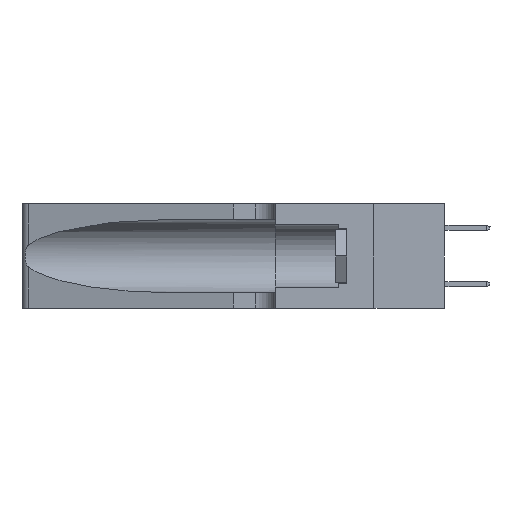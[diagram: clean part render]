
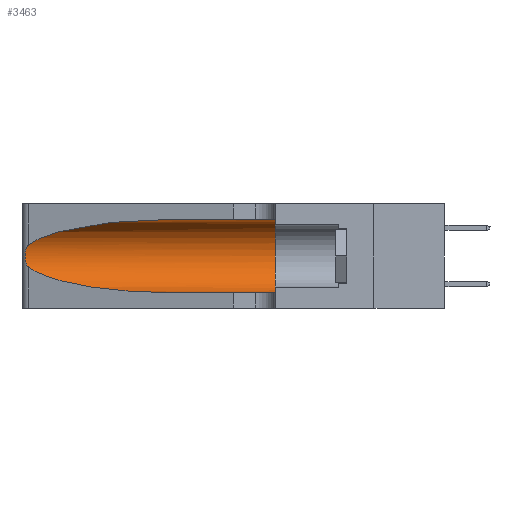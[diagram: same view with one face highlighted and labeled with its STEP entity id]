
A CAD part, left-side view. The second image highlights one B-rep face of the part: STEP entity #3463.
In plain terms, the highlighted cylindrical face has radius 3.308 mm (diameter 6.617 mm), a partial arc.
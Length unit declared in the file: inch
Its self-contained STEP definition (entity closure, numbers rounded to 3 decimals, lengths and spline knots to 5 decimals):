
#256 = CARTESIAN_POINT ( 'NONE',  ( 0.1305, 1.61858, 0.31525 ) ) ;
#488 = VERTEX_POINT ( 'NONE', #8735 ) ;
#558 = DIRECTION ( 'NONE',  ( 0., 0., -1. ) ) ;
#919 = CARTESIAN_POINT ( 'NONE',  ( 0.25639, 1.23184, 0.21858 ) ) ;
#1046 = CARTESIAN_POINT ( 'NONE',  ( 0.26017, 1.23833, 0.17102 ) ) ;
#1629 = DIRECTION ( 'NONE',  ( 0., 1., 0. ) ) ;
#1738 = CARTESIAN_POINT ( 'NONE',  ( 0.1305, 0.72297, 0.05475 ) ) ;
#2156 = CARTESIAN_POINT ( 'NONE',  ( 0.18966, 0.96281, 0.05475 ) ) ;
#2170 = ORIENTED_EDGE ( 'NONE', *, *, #7183, .T. ) ;
#2276 = CARTESIAN_POINT ( 'NONE',  ( 0.25789, 1.23486, 0.15765 ) ) ;
#2587 = VECTOR ( 'NONE', #6067, 39.37008 ) ;
#2995 = CARTESIAN_POINT ( 'NONE',  ( 0.25487, 1.22718, 0.22369 ) ) ;
#3277 = VECTOR ( 'NONE', #17913, 39.37008 ) ;
#3463 = ADVANCED_FACE ( 'NONE', ( #11032 ), #7582, .F. ) ;
#3469 = ORIENTED_EDGE ( 'NONE', *, *, #18091, .T. ) ;
#3883 = CARTESIAN_POINT ( 'NONE',  ( 0.25639, 1.23186, 0.15144 ) ) ;
#4797 = AXIS2_PLACEMENT_3D ( 'NONE', #17805, #1629, #17873 ) ;
#5348 = LINE ( 'NONE', #14806, #2587 ) ;
#6005 = LINE ( 'NONE', #256, #3277 ) ;
#6067 = DIRECTION ( 'NONE',  ( 0., -1., 0. ) ) ;
#6241 = EDGE_LOOP ( 'NONE', ( #17722, #2170, #3469, #12455, #13920, #12567 ) ) ;
#6276 = CARTESIAN_POINT ( 'NONE',  ( 0.1305, 1.61858, 0.185 ) ) ;
#6574 = CARTESIAN_POINT ( 'NONE',  ( 0.1305, 0.72297, 0.05475 ) ) ;
#6628 = CARTESIAN_POINT ( 'NONE',  ( 0.26018, 1.23835, 0.19895 ) ) ;
#6645 = VERTEX_POINT ( 'NONE', #17974 ) ;
#6747 = CARTESIAN_POINT ( 'NONE',  ( 0.25854, 1.2359, 0.20912 ) ) ;
#7183 = EDGE_CURVE ( 'NONE', #8647, #6645, #15826, .T. ) ;
#7582 = CYLINDRICAL_SURFACE ( 'NONE', #13383, 0.13025 ) ;
#7894 = EDGE_CURVE ( 'NONE', #15827, #8647, #16660, .T. ) ;
#8082 = CARTESIAN_POINT ( 'NONE',  ( 0.25487, 1.22718, 0.22369 ) ) ;
#8459 = CARTESIAN_POINT ( 'NONE',  ( 0.18966, 0.96281, 0.31525 ) ) ;
#8647 = VERTEX_POINT ( 'NONE', #2995 ) ;
#8735 = CARTESIAN_POINT ( 'NONE',  ( 0.1305, 0.35, 0.05475 ) ) ;
#8781 =( BOUNDED_CURVE ( )  B_SPLINE_CURVE ( 3, ( #12765, #17136, #2156, #6574 ),
 .UNSPECIFIED., .F., .F. ) 
 B_SPLINE_CURVE_WITH_KNOTS ( ( 4, 4 ),
 ( 3.44316, 4.71239 ),
 .UNSPECIFIED. ) 
 CURVE ( )  GEOMETRIC_REPRESENTATION_ITEM ( )  RATIONAL_B_SPLINE_CURVE ( ( 1., 0.87, 0.87, 1. ) ) 
 REPRESENTATION_ITEM ( '' )  );
#9706 = EDGE_CURVE ( 'NONE', #15827, #12617, #6005, .T. ) ;
#9782 = CARTESIAN_POINT ( 'NONE',  ( 0.1305, 0.72297, 0.31525 ) ) ;
#9786 = CARTESIAN_POINT ( 'NONE',  ( 0.25487, 1.22718, 0.14631 ) ) ;
#11032 = FACE_OUTER_BOUND ( 'NONE', #6241, .T. ) ;
#11165 = CARTESIAN_POINT ( 'NONE',  ( 0.25856, 1.23593, 0.16098 ) ) ;
#11533 = CARTESIAN_POINT ( 'NONE',  ( 0.2373, 1.15595, 0.28018 ) ) ;
#12455 = ORIENTED_EDGE ( 'NONE', *, *, #15504, .T. ) ;
#12567 = ORIENTED_EDGE ( 'NONE', *, *, #9706, .F. ) ;
#12617 = VERTEX_POINT ( 'NONE', #13093 ) ;
#12765 = CARTESIAN_POINT ( 'NONE',  ( 0.25487, 1.22718, 0.14631 ) ) ;
#13093 = CARTESIAN_POINT ( 'NONE',  ( 0.1305, 0.35, 0.31525 ) ) ;
#13171 = EDGE_CURVE ( 'NONE', #12617, #488, #18221, .T. ) ;
#13383 = AXIS2_PLACEMENT_3D ( 'NONE', #6276, #16561, #558 ) ;
#13920 = ORIENTED_EDGE ( 'NONE', *, *, #13171, .F. ) ;
#14806 = CARTESIAN_POINT ( 'NONE',  ( 0.1305, 1.61858, 0.05475 ) ) ;
#15211 = VERTEX_POINT ( 'NONE', #1738 ) ;
#15376 = CARTESIAN_POINT ( 'NONE',  ( 0.25555, 1.22994, 0.2215 ) ) ;
#15503 = CARTESIAN_POINT ( 'NONE',  ( 0.25787, 1.23484, 0.2124 ) ) ;
#15504 = EDGE_CURVE ( 'NONE', #15211, #488, #5348, .T. ) ;
#15826 = B_SPLINE_CURVE_WITH_KNOTS ( 'NONE', 3,
 ( #8082, #15376, #919, #15503, #6747, #6628, #16993, #18325, #1046, #11165, #2276, #3883, #17116, #9786 ),
 .UNSPECIFIED., .F., .F.,
 ( 4, 2, 2, 2, 2, 2, 4 ),
 ( 0., 0.00027, 0.00053, 0.00107, 0.0016, 0.00187, 0.00214 ),
 .UNSPECIFIED. ) ;
#15827 = VERTEX_POINT ( 'NONE', #18068 ) ;
#16561 = DIRECTION ( 'NONE',  ( 0., -1., 0. ) ) ;
#16660 =( BOUNDED_CURVE ( )  B_SPLINE_CURVE ( 3, ( #9782, #8459, #11533, #18692 ),
 .UNSPECIFIED., .F., .F. ) 
 B_SPLINE_CURVE_WITH_KNOTS ( ( 4, 4 ),
 ( 1.5708, 2.84003 ),
 .UNSPECIFIED. ) 
 CURVE ( )  GEOMETRIC_REPRESENTATION_ITEM ( )  RATIONAL_B_SPLINE_CURVE ( ( 1., 0.87, 0.87, 1. ) ) 
 REPRESENTATION_ITEM ( '' )  );
#16993 = CARTESIAN_POINT ( 'NONE',  ( 0.26075, 1.23896, 0.19203 ) ) ;
#17116 = CARTESIAN_POINT ( 'NONE',  ( 0.25555, 1.22993, 0.14849 ) ) ;
#17136 = CARTESIAN_POINT ( 'NONE',  ( 0.2373, 1.15595, 0.08982 ) ) ;
#17722 = ORIENTED_EDGE ( 'NONE', *, *, #7894, .T. ) ;
#17805 = CARTESIAN_POINT ( 'NONE',  ( 0.1305, 0.35, 0.185 ) ) ;
#17873 = DIRECTION ( 'NONE',  ( 0., 0., 1. ) ) ;
#17913 = DIRECTION ( 'NONE',  ( 0., -1., 0. ) ) ;
#17974 = CARTESIAN_POINT ( 'NONE',  ( 0.25487, 1.22718, 0.14631 ) ) ;
#18068 = CARTESIAN_POINT ( 'NONE',  ( 0.1305, 0.72297, 0.31525 ) ) ;
#18091 = EDGE_CURVE ( 'NONE', #6645, #15211, #8781, .T. ) ;
#18221 = CIRCLE ( 'NONE', #4797, 0.13025 ) ;
#18325 = CARTESIAN_POINT ( 'NONE',  ( 0.26075, 1.23896, 0.178 ) ) ;
#18692 = CARTESIAN_POINT ( 'NONE',  ( 0.25487, 1.22718, 0.22369 ) ) ;
